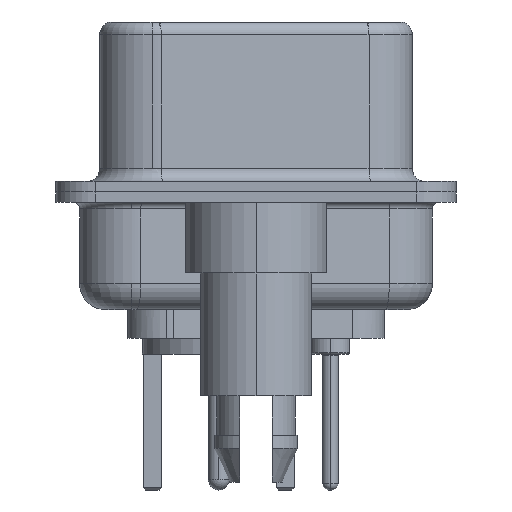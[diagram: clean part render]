
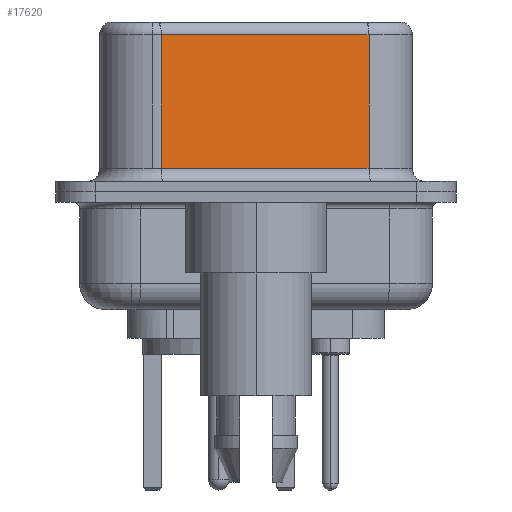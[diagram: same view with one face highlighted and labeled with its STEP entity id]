
A CAD part, left-side view. The second image highlights one B-rep face of the part: STEP entity #17620.
In plain terms, the highlighted planar face has unit normal (-0.985, -0.174, 0).
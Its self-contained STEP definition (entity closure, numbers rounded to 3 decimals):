
#22 = CARTESIAN_POINT ( 'NONE',  ( 5.132, -4.322, 0.9 ) ) ;
#32 = VECTOR ( 'NONE', #20123, 1000. ) ;
#978 = DIRECTION ( 'NONE',  ( 0., 0., -1. ) ) ;
#1016 = ORIENTED_EDGE ( 'NONE', *, *, #4307, .T. ) ;
#1207 = CARTESIAN_POINT ( 'NONE',  ( 5.132, -4.322, 6.52 ) ) ;
#1294 = PLANE ( 'NONE',  #9373 ) ;
#2228 = CARTESIAN_POINT ( 'NONE',  ( 3.73, 3.628, 6.52 ) ) ;
#2492 = ORIENTED_EDGE ( 'NONE', *, *, #8768, .F. ) ;
#2979 = VECTOR ( 'NONE', #978, 1000. ) ;
#4027 = CARTESIAN_POINT ( 'NONE',  ( 5.132, -4.322, 6.02 ) ) ;
#4091 = DIRECTION ( 'NONE',  ( -0.174, 0.985, 0. ) ) ;
#4307 = EDGE_CURVE ( 'NONE', #18518, #8915, #11635, .T. ) ;
#4526 = CARTESIAN_POINT ( 'NONE',  ( 5.132, -4.322, 0.9 ) ) ;
#4686 = VECTOR ( 'NONE', #9529, 1000. ) ;
#4755 = ORIENTED_EDGE ( 'NONE', *, *, #26552, .T. ) ;
#6209 = LINE ( 'NONE', #4526, #32 ) ;
#8598 = EDGE_CURVE ( 'NONE', #23064, #18518, #18442, .T. ) ;
#8768 = EDGE_CURVE ( 'NONE', #23064, #25953, #8962, .T. ) ;
#8915 = VERTEX_POINT ( 'NONE', #24561 ) ;
#8962 = LINE ( 'NONE', #1207, #2979 ) ;
#9373 = AXIS2_PLACEMENT_3D ( 'NONE', #19333, #23719, #10419 ) ;
#9529 = DIRECTION ( 'NONE',  ( 0., 0., -1. ) ) ;
#10419 = DIRECTION ( 'NONE',  ( -0.174, 0.985, 0. ) ) ;
#11635 = LINE ( 'NONE', #2228, #4686 ) ;
#11934 = CARTESIAN_POINT ( 'NONE',  ( 5.132, -4.322, 6.02 ) ) ;
#12507 = VECTOR ( 'NONE', #4091, 1000. ) ;
#14932 = FACE_OUTER_BOUND ( 'NONE', #27545, .T. ) ;
#17620 = ADVANCED_FACE ( 'NONE', ( #14932 ), #1294, .F. ) ;
#18064 = ORIENTED_EDGE ( 'NONE', *, *, #8598, .T. ) ;
#18442 = LINE ( 'NONE', #4027, #12507 ) ;
#18518 = VERTEX_POINT ( 'NONE', #26399 ) ;
#19333 = CARTESIAN_POINT ( 'NONE',  ( 5.132, -4.322, 6.52 ) ) ;
#20123 = DIRECTION ( 'NONE',  ( 0.174, -0.985, 0. ) ) ;
#23064 = VERTEX_POINT ( 'NONE', #11934 ) ;
#23719 = DIRECTION ( 'NONE',  ( 0.985, 0.174, 0. ) ) ;
#24561 = CARTESIAN_POINT ( 'NONE',  ( 3.73, 3.628, 0.9 ) ) ;
#25953 = VERTEX_POINT ( 'NONE', #22 ) ;
#26399 = CARTESIAN_POINT ( 'NONE',  ( 3.73, 3.628, 6.02 ) ) ;
#26552 = EDGE_CURVE ( 'NONE', #8915, #25953, #6209, .T. ) ;
#27545 = EDGE_LOOP ( 'NONE', ( #2492, #18064, #1016, #4755 ) ) ;
